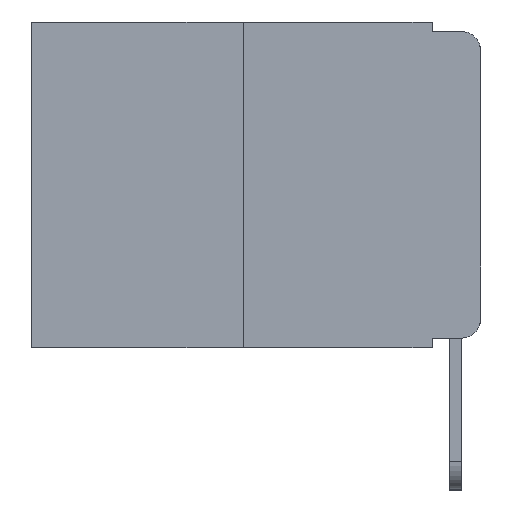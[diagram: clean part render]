
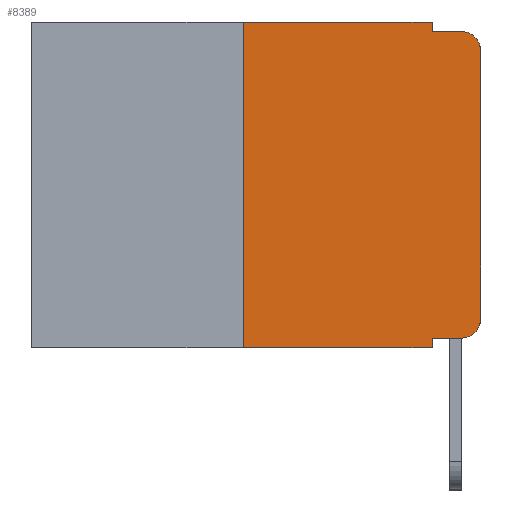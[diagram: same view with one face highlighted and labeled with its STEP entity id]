
A CAD part, left-side view. The second image highlights one B-rep face of the part: STEP entity #8389.
In plain terms, the highlighted planar face has unit normal (-1, 0, 0).
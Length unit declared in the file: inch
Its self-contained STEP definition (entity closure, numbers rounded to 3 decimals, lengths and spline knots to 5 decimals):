
#124 = ORIENTED_EDGE ( 'NONE', *, *, #15610, .T. ) ;
#613 = LINE ( 'NONE', #6410, #10532 ) ;
#1054 = LINE ( 'NONE', #8609, #9273 ) ;
#1366 = DIRECTION ( 'NONE',  ( 0., 0., 1. ) ) ;
#1420 = CIRCLE ( 'NONE', #12376, 0.02 ) ;
#1426 = CARTESIAN_POINT ( 'NONE',  ( 0., 0.051, -0.01 ) ) ;
#1433 = DIRECTION ( 'NONE',  ( 1., 0., 0. ) ) ;
#1638 = DIRECTION ( 'NONE',  ( 0., 0., -1. ) ) ;
#2529 = ORIENTED_EDGE ( 'NONE', *, *, #17631, .T. ) ;
#2545 = ORIENTED_EDGE ( 'NONE', *, *, #18380, .F. ) ;
#2730 = EDGE_CURVE ( 'NONE', #3292, #13042, #2902, .T. ) ;
#2902 = LINE ( 'NONE', #8563, #13257 ) ;
#3013 = DIRECTION ( 'NONE',  ( 0., -1., 0. ) ) ;
#3159 = CARTESIAN_POINT ( 'NONE',  ( 0., 0., 0. ) ) ;
#3292 = VERTEX_POINT ( 'NONE', #13430 ) ;
#3392 = EDGE_CURVE ( 'NONE', #15645, #13388, #1420, .T. ) ;
#3472 = VERTEX_POINT ( 'NONE', #1426 ) ;
#3493 = DIRECTION ( 'NONE',  ( 0., -1., 0. ) ) ;
#3497 = VERTEX_POINT ( 'NONE', #15844 ) ;
#3552 = DIRECTION ( 'NONE',  ( -1., 0., 0. ) ) ;
#3664 = CARTESIAN_POINT ( 'NONE',  ( 0., 0.051, 0. ) ) ;
#4099 = VECTOR ( 'NONE', #18510, 39.37008 ) ;
#4113 = CARTESIAN_POINT ( 'NONE',  ( 0., 0.051, 0. ) ) ;
#4283 = EDGE_CURVE ( 'NONE', #16118, #3472, #11086, .T. ) ;
#4398 = CARTESIAN_POINT ( 'NONE',  ( 0., 0.473, 0. ) ) ;
#5115 = DIRECTION ( 'NONE',  ( 0., 0., -1. ) ) ;
#5142 = DIRECTION ( 'NONE',  ( 0., 0., -1. ) ) ;
#5308 = EDGE_LOOP ( 'NONE', ( #2529, #15550, #15370, #14086, #12375, #8594, #124, #2545, #15086, #13288 ) ) ;
#5719 = EDGE_CURVE ( 'NONE', #12069, #15645, #15286, .T. ) ;
#5747 = FACE_OUTER_BOUND ( 'NONE', #5308, .T. ) ;
#5832 = CARTESIAN_POINT ( 'NONE',  ( 0., 0.473, 0. ) ) ;
#6212 = VECTOR ( 'NONE', #5142, 39.37008 ) ;
#6410 = CARTESIAN_POINT ( 'NONE',  ( 0., 0.473, -0.343 ) ) ;
#6506 = EDGE_CURVE ( 'NONE', #3472, #3497, #6567, .T. ) ;
#6567 = LINE ( 'NONE', #13717, #4099 ) ;
#8389 = ADVANCED_FACE ( 'NONE', ( #5747 ), #13294, .F. ) ;
#8563 = CARTESIAN_POINT ( 'NONE',  ( 0., 0.25, 0. ) ) ;
#8594 = ORIENTED_EDGE ( 'NONE', *, *, #2730, .F. ) ;
#8609 = CARTESIAN_POINT ( 'NONE',  ( 0., 0.051, 0. ) ) ;
#9273 = VECTOR ( 'NONE', #15936, 39.37008 ) ;
#9781 = CARTESIAN_POINT ( 'NONE',  ( 0., 0.02, -0.313 ) ) ;
#9852 = CARTESIAN_POINT ( 'NONE',  ( 0., 0.051, -0.333 ) ) ;
#10532 = VECTOR ( 'NONE', #3493, 39.37008 ) ;
#10592 = CARTESIAN_POINT ( 'NONE',  ( 0., 0.25, 0. ) ) ;
#10668 = LINE ( 'NONE', #3159, #13011 ) ;
#11086 = LINE ( 'NONE', #3664, #6212 ) ;
#12069 = VERTEX_POINT ( 'NONE', #9852 ) ;
#12253 = DIRECTION ( 'NONE',  ( 0., -1., 0. ) ) ;
#12375 = ORIENTED_EDGE ( 'NONE', *, *, #16537, .F. ) ;
#12376 = AXIS2_PLACEMENT_3D ( 'NONE', #9781, #3552, #5115 ) ;
#12891 = AXIS2_PLACEMENT_3D ( 'NONE', #4398, #1433, #1638 ) ;
#13011 = VECTOR ( 'NONE', #1366, 39.37008 ) ;
#13042 = VERTEX_POINT ( 'NONE', #10592 ) ;
#13132 = CARTESIAN_POINT ( 'NONE',  ( 0., 0., -0.03 ) ) ;
#13171 = LINE ( 'NONE', #5832, #18926 ) ;
#13257 = VECTOR ( 'NONE', #14512, 39.37008 ) ;
#13288 = ORIENTED_EDGE ( 'NONE', *, *, #3392, .T. ) ;
#13294 = PLANE ( 'NONE',  #12891 ) ;
#13388 = VERTEX_POINT ( 'NONE', #17527 ) ;
#13430 = CARTESIAN_POINT ( 'NONE',  ( 0., 0.25, -0.343 ) ) ;
#13449 = VECTOR ( 'NONE', #12253, 39.37008 ) ;
#13717 = CARTESIAN_POINT ( 'NONE',  ( 0., 0.051, -0.01 ) ) ;
#13925 = DIRECTION ( 'NONE',  ( 0., 0., -1. ) ) ;
#14086 = ORIENTED_EDGE ( 'NONE', *, *, #4283, .F. ) ;
#14196 = DIRECTION ( 'NONE',  ( -1., 0., 0. ) ) ;
#14223 = CIRCLE ( 'NONE', #19245, 0.02 ) ;
#14512 = DIRECTION ( 'NONE',  ( 0., 0., 1. ) ) ;
#14919 = CARTESIAN_POINT ( 'NONE',  ( 0., 0.051, -0.343 ) ) ;
#15086 = ORIENTED_EDGE ( 'NONE', *, *, #5719, .T. ) ;
#15286 = LINE ( 'NONE', #16754, #13449 ) ;
#15370 = ORIENTED_EDGE ( 'NONE', *, *, #6506, .F. ) ;
#15550 = ORIENTED_EDGE ( 'NONE', *, *, #17290, .T. ) ;
#15568 = CARTESIAN_POINT ( 'NONE',  ( 0., 0.02, -0.03 ) ) ;
#15610 = EDGE_CURVE ( 'NONE', #3292, #16749, #613, .T. ) ;
#15645 = VERTEX_POINT ( 'NONE', #18447 ) ;
#15844 = CARTESIAN_POINT ( 'NONE',  ( 0., 0.02, -0.01 ) ) ;
#15936 = DIRECTION ( 'NONE',  ( 0., 0., -1. ) ) ;
#16118 = VERTEX_POINT ( 'NONE', #4113 ) ;
#16537 = EDGE_CURVE ( 'NONE', #13042, #16118, #13171, .T. ) ;
#16749 = VERTEX_POINT ( 'NONE', #14919 ) ;
#16754 = CARTESIAN_POINT ( 'NONE',  ( 0., 0.051, -0.333 ) ) ;
#17290 = EDGE_CURVE ( 'NONE', #17499, #3497, #14223, .T. ) ;
#17499 = VERTEX_POINT ( 'NONE', #13132 ) ;
#17527 = CARTESIAN_POINT ( 'NONE',  ( 0., 0., -0.313 ) ) ;
#17631 = EDGE_CURVE ( 'NONE', #13388, #17499, #10668, .T. ) ;
#18380 = EDGE_CURVE ( 'NONE', #12069, #16749, #1054, .T. ) ;
#18447 = CARTESIAN_POINT ( 'NONE',  ( 0., 0.02, -0.333 ) ) ;
#18510 = DIRECTION ( 'NONE',  ( 0., -1., 0. ) ) ;
#18926 = VECTOR ( 'NONE', #3013, 39.37008 ) ;
#19245 = AXIS2_PLACEMENT_3D ( 'NONE', #15568, #14196, #13925 ) ;
